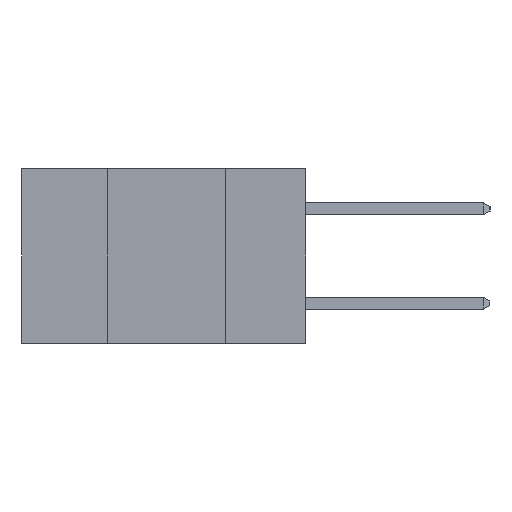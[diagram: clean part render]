
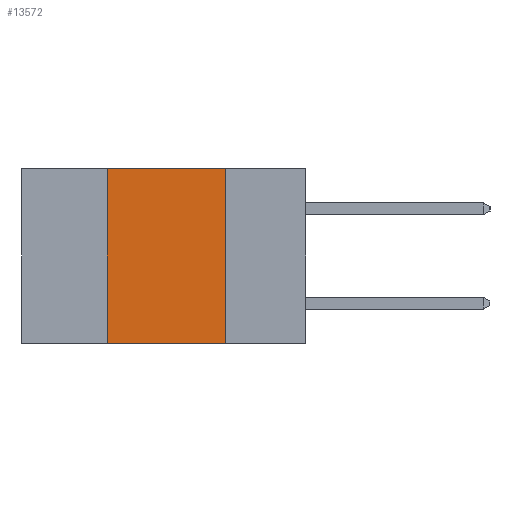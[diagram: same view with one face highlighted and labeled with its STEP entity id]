
A CAD part, left-side view. The second image highlights one B-rep face of the part: STEP entity #13572.
In plain terms, the highlighted planar face has unit normal (-1, 0, 0).
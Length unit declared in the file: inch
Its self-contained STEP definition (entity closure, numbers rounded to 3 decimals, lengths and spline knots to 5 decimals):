
#1301 = DIRECTION ( 'NONE',  ( 0., 0., -1. ) ) ;
#1488 = VECTOR ( 'NONE', #1301, 39.37008 ) ;
#2201 = DIRECTION ( 'NONE',  ( 1., 0., 0. ) ) ;
#4153 = ORIENTED_EDGE ( 'NONE', *, *, #13017, .F. ) ;
#4187 = FACE_OUTER_BOUND ( 'NONE', #20704, .T. ) ;
#6154 = CARTESIAN_POINT ( 'NONE',  ( 0., 0.42, -0.37 ) ) ;
#6849 = VERTEX_POINT ( 'NONE', #9379 ) ;
#7559 = ORIENTED_EDGE ( 'NONE', *, *, #18189, .F. ) ;
#7720 = CARTESIAN_POINT ( 'NONE',  ( 0., 0.42, 0. ) ) ;
#7790 = LINE ( 'NONE', #22057, #13263 ) ;
#8474 = LINE ( 'NONE', #13596, #11379 ) ;
#8763 = VERTEX_POINT ( 'NONE', #7720 ) ;
#8994 = CARTESIAN_POINT ( 'NONE',  ( 0., 0.6, 0. ) ) ;
#9379 = CARTESIAN_POINT ( 'NONE',  ( 0., 0.17, -0.37 ) ) ;
#10418 = EDGE_CURVE ( 'NONE', #20738, #6849, #17325, .T. ) ;
#11150 = EDGE_CURVE ( 'NONE', #14106, #6849, #8474, .T. ) ;
#11198 = PLANE ( 'NONE',  #11767 ) ;
#11379 = VECTOR ( 'NONE', #11624, 39.37008 ) ;
#11624 = DIRECTION ( 'NONE',  ( 0., -1., 0. ) ) ;
#11767 = AXIS2_PLACEMENT_3D ( 'NONE', #12821, #2201, #16566 ) ;
#12821 = CARTESIAN_POINT ( 'NONE',  ( 0., 0.6, 0. ) ) ;
#13017 = EDGE_CURVE ( 'NONE', #14106, #8763, #7790, .T. ) ;
#13263 = VECTOR ( 'NONE', #13492, 39.37008 ) ;
#13492 = DIRECTION ( 'NONE',  ( 0., 0., 1. ) ) ;
#13572 = ADVANCED_FACE ( 'NONE', ( #4187 ), #11198, .F. ) ;
#13596 = CARTESIAN_POINT ( 'NONE',  ( 0., 0.6, -0.37 ) ) ;
#14106 = VERTEX_POINT ( 'NONE', #6154 ) ;
#14348 = LINE ( 'NONE', #8994, #16756 ) ;
#15228 = CARTESIAN_POINT ( 'NONE',  ( 0., 0.17, 0. ) ) ;
#16566 = DIRECTION ( 'NONE',  ( 0., 0., -1. ) ) ;
#16756 = VECTOR ( 'NONE', #21726, 39.37008 ) ;
#17325 = LINE ( 'NONE', #22712, #1488 ) ;
#18189 = EDGE_CURVE ( 'NONE', #8763, #20738, #14348, .T. ) ;
#19015 = ORIENTED_EDGE ( 'NONE', *, *, #10418, .F. ) ;
#20704 = EDGE_LOOP ( 'NONE', ( #19015, #7559, #4153, #23069 ) ) ;
#20738 = VERTEX_POINT ( 'NONE', #15228 ) ;
#21726 = DIRECTION ( 'NONE',  ( 0., -1., 0. ) ) ;
#22057 = CARTESIAN_POINT ( 'NONE',  ( 0., 0.42, -0.37 ) ) ;
#22712 = CARTESIAN_POINT ( 'NONE',  ( 0., 0.17, -0.37 ) ) ;
#23069 = ORIENTED_EDGE ( 'NONE', *, *, #11150, .T. ) ;
